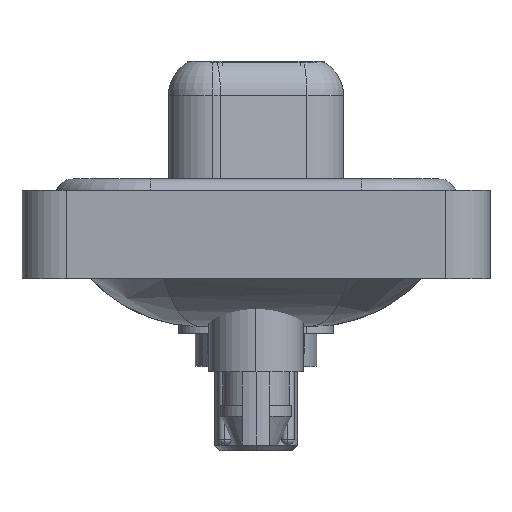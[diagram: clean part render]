
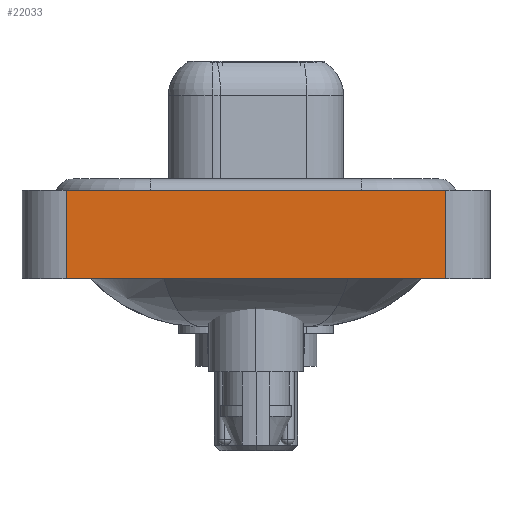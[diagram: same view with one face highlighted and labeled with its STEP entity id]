
A CAD part, left-side view. The second image highlights one B-rep face of the part: STEP entity #22033.
In plain terms, the highlighted planar face has unit normal (-1, 0, 0).
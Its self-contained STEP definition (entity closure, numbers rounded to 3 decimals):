
#1032 = VECTOR ( 'NONE', #7495, 1000. ) ;
#1736 = VECTOR ( 'NONE', #18810, 1000. ) ;
#1964 = CARTESIAN_POINT ( 'NONE',  ( -7.3, -8.55, -3.6 ) ) ;
#2657 = VERTEX_POINT ( 'NONE', #22546 ) ;
#3441 = CARTESIAN_POINT ( 'NONE',  ( -7.3, 8.55, -3.6 ) ) ;
#3457 = EDGE_CURVE ( 'NONE', #2657, #23348, #20302, .T. ) ;
#5137 = CARTESIAN_POINT ( 'NONE',  ( -7.3, -8.55, 0.4 ) ) ;
#5200 = VECTOR ( 'NONE', #14822, 1000. ) ;
#5414 = EDGE_CURVE ( 'NONE', #23274, #2657, #13014, .T. ) ;
#5782 = EDGE_CURVE ( 'NONE', #23274, #12273, #8125, .T. ) ;
#6795 = CARTESIAN_POINT ( 'NONE',  ( -7.3, -8.55, -3.6 ) ) ;
#7495 = DIRECTION ( 'NONE',  ( 0., -1., 0. ) ) ;
#8125 = LINE ( 'NONE', #18924, #1736 ) ;
#8622 = LINE ( 'NONE', #5137, #1032 ) ;
#9028 = ORIENTED_EDGE ( 'NONE', *, *, #14628, .F. ) ;
#10205 = EDGE_LOOP ( 'NONE', ( #23665, #9028, #10981, #15841 ) ) ;
#10981 = ORIENTED_EDGE ( 'NONE', *, *, #5782, .F. ) ;
#11305 = DIRECTION ( 'NONE',  ( 0., 0., 1. ) ) ;
#12273 = VERTEX_POINT ( 'NONE', #22111 ) ;
#13014 = LINE ( 'NONE', #1964, #5200 ) ;
#14119 = DIRECTION ( 'NONE',  ( -1., 0., 0. ) ) ;
#14628 = EDGE_CURVE ( 'NONE', #12273, #23348, #8622, .T. ) ;
#14822 = DIRECTION ( 'NONE',  ( 0., -1., 0. ) ) ;
#15841 = ORIENTED_EDGE ( 'NONE', *, *, #5414, .T. ) ;
#16509 = CARTESIAN_POINT ( 'NONE',  ( -7.3, -8.55, 0.4 ) ) ;
#17595 = PLANE ( 'NONE',  #20702 ) ;
#18810 = DIRECTION ( 'NONE',  ( 0., 0., 1. ) ) ;
#18924 = CARTESIAN_POINT ( 'NONE',  ( -7.3, 8.55, -3.6 ) ) ;
#19342 = VECTOR ( 'NONE', #11305, 1000. ) ;
#19881 = FACE_OUTER_BOUND ( 'NONE', #10205, .T. ) ;
#20302 = LINE ( 'NONE', #22463, #19342 ) ;
#20702 = AXIS2_PLACEMENT_3D ( 'NONE', #6795, #14119, #21445 ) ;
#21445 = DIRECTION ( 'NONE',  ( 0., 0., 1. ) ) ;
#22033 = ADVANCED_FACE ( 'NONE', ( #19881 ), #17595, .T. ) ;
#22111 = CARTESIAN_POINT ( 'NONE',  ( -7.3, 8.55, 0.4 ) ) ;
#22463 = CARTESIAN_POINT ( 'NONE',  ( -7.3, -8.55, -3.6 ) ) ;
#22546 = CARTESIAN_POINT ( 'NONE',  ( -7.3, -8.55, -3.6 ) ) ;
#23274 = VERTEX_POINT ( 'NONE', #3441 ) ;
#23348 = VERTEX_POINT ( 'NONE', #16509 ) ;
#23665 = ORIENTED_EDGE ( 'NONE', *, *, #3457, .T. ) ;
